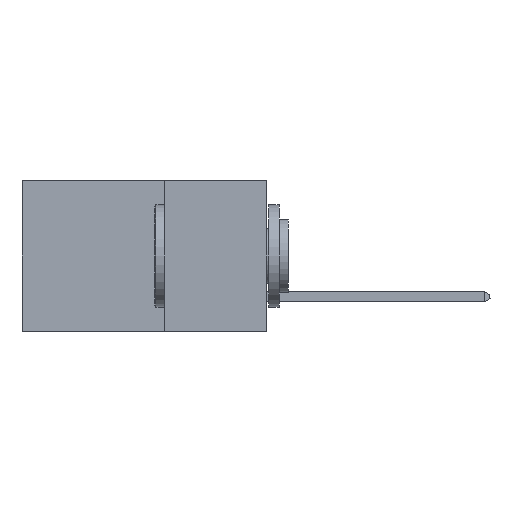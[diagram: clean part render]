
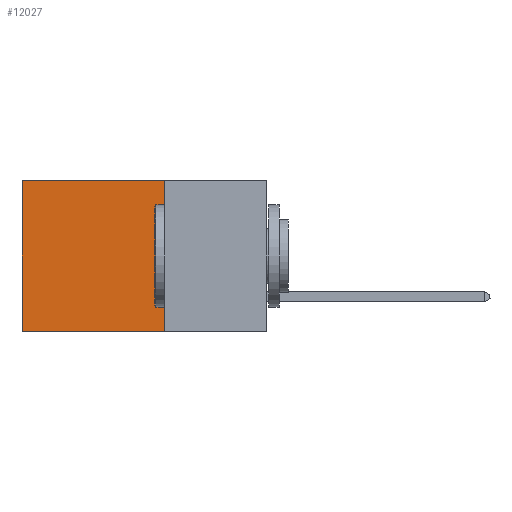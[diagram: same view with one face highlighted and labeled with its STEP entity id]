
A CAD part, left-side view. The second image highlights one B-rep face of the part: STEP entity #12027.
In plain terms, the highlighted planar face has unit normal (-1, 0, 0).
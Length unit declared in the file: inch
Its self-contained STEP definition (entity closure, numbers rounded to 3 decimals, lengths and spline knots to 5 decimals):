
#397 = VERTEX_POINT ( 'NONE', #1734 ) ;
#548 = EDGE_LOOP ( 'NONE', ( #10960, #7945, #1418, #13243 ) ) ;
#1174 = LINE ( 'NONE', #1478, #11163 ) ;
#1296 = VECTOR ( 'NONE', #5764, 39.37008 ) ;
#1418 = ORIENTED_EDGE ( 'NONE', *, *, #9871, .F. ) ;
#1478 = CARTESIAN_POINT ( 'NONE',  ( 0.2875, 0.25, 0. ) ) ;
#1734 = CARTESIAN_POINT ( 'NONE',  ( 0.2875, 0.6, 0. ) ) ;
#1746 = EDGE_CURVE ( 'NONE', #397, #10784, #14122, .T. ) ;
#1817 = CARTESIAN_POINT ( 'NONE',  ( 0.2875, 0.25, -0.37 ) ) ;
#2652 = EDGE_CURVE ( 'NONE', #3605, #397, #8685, .T. ) ;
#2661 = DIRECTION ( 'NONE',  ( 0., 0., -1. ) ) ;
#2952 = EDGE_CURVE ( 'NONE', #13921, #10784, #7974, .T. ) ;
#3430 = CARTESIAN_POINT ( 'NONE',  ( 0.2875, 0.6, 0. ) ) ;
#3605 = VERTEX_POINT ( 'NONE', #6817 ) ;
#4134 = DIRECTION ( 'NONE',  ( 0., 0., -1. ) ) ;
#4609 = CARTESIAN_POINT ( 'NONE',  ( 0.2875, 0.25, 0. ) ) ;
#4872 = CARTESIAN_POINT ( 'NONE',  ( 0.2875, 0.6, -0.37 ) ) ;
#5214 = PLANE ( 'NONE',  #11424 ) ;
#5636 = FACE_OUTER_BOUND ( 'NONE', #548, .T. ) ;
#5764 = DIRECTION ( 'NONE',  ( 0., 1., 0. ) ) ;
#6817 = CARTESIAN_POINT ( 'NONE',  ( 0.2875, 0.25, 0. ) ) ;
#7292 = DIRECTION ( 'NONE',  ( 0., 1., 0. ) ) ;
#7821 = VECTOR ( 'NONE', #7292, 39.37008 ) ;
#7945 = ORIENTED_EDGE ( 'NONE', *, *, #2952, .F. ) ;
#7974 = LINE ( 'NONE', #1817, #7821 ) ;
#8685 = LINE ( 'NONE', #4609, #1296 ) ;
#9120 = DIRECTION ( 'NONE',  ( 0., 0., -1. ) ) ;
#9396 = VECTOR ( 'NONE', #9120, 39.37008 ) ;
#9600 = CARTESIAN_POINT ( 'NONE',  ( 0.2875, 0.25, -0.37 ) ) ;
#9871 = EDGE_CURVE ( 'NONE', #3605, #13921, #1174, .T. ) ;
#10784 = VERTEX_POINT ( 'NONE', #4872 ) ;
#10960 = ORIENTED_EDGE ( 'NONE', *, *, #1746, .T. ) ;
#11163 = VECTOR ( 'NONE', #2661, 39.37008 ) ;
#11424 = AXIS2_PLACEMENT_3D ( 'NONE', #12946, #12993, #4134 ) ;
#12027 = ADVANCED_FACE ( 'NONE', ( #5636 ), #5214, .F. ) ;
#12946 = CARTESIAN_POINT ( 'NONE',  ( 0.2875, 0.25, 0. ) ) ;
#12993 = DIRECTION ( 'NONE',  ( 1., 0., 0. ) ) ;
#13243 = ORIENTED_EDGE ( 'NONE', *, *, #2652, .T. ) ;
#13921 = VERTEX_POINT ( 'NONE', #9600 ) ;
#14122 = LINE ( 'NONE', #3430, #9396 ) ;
